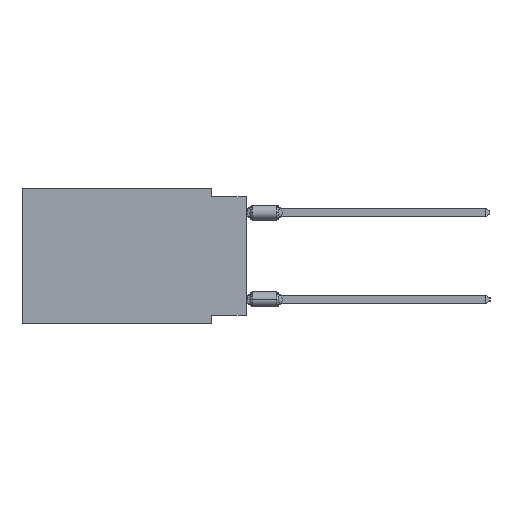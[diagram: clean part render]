
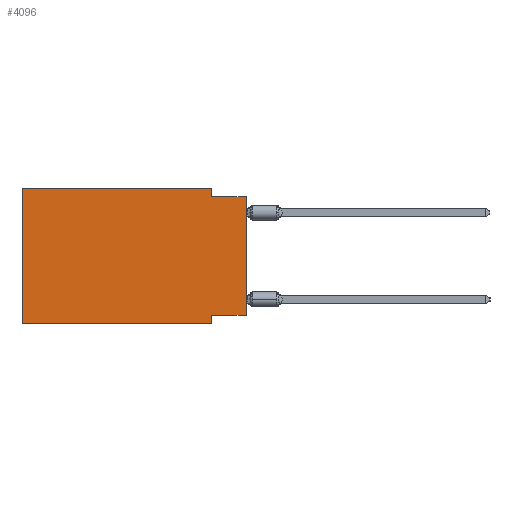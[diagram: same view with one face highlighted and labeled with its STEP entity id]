
A CAD part, left-side view. The second image highlights one B-rep face of the part: STEP entity #4096.
In plain terms, the highlighted planar face has unit normal (-1, 0, 0).
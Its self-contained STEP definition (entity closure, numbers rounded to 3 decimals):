
#33 = CARTESIAN_POINT ( 'NONE',  ( 0., 2.54, -0.635 ) ) ;
#934 = AXIS2_PLACEMENT_3D ( 'NONE', #39811, #10003, #10648 ) ;
#1196 = LINE ( 'NONE', #40220, #36049 ) ;
#1212 = VECTOR ( 'NONE', #21840, 1000. ) ;
#1689 = EDGE_CURVE ( 'NONE', #2483, #50379, #26597, .T. ) ;
#2483 = VERTEX_POINT ( 'NONE', #11028 ) ;
#2522 = EDGE_CURVE ( 'NONE', #21431, #20861, #62807, .T. ) ;
#4096 = ADVANCED_FACE ( 'NONE', ( #26387 ), #54907, .F. ) ;
#5152 = ORIENTED_EDGE ( 'NONE', *, *, #10090, .F. ) ;
#5382 = ORIENTED_EDGE ( 'NONE', *, *, #25717, .F. ) ;
#5768 = VERTEX_POINT ( 'NONE', #33 ) ;
#5859 = EDGE_CURVE ( 'NONE', #32394, #39374, #56073, .T. ) ;
#6676 = VERTEX_POINT ( 'NONE', #11914 ) ;
#7737 = CARTESIAN_POINT ( 'NONE',  ( 0., 16.383, 0. ) ) ;
#10003 = DIRECTION ( 'NONE',  ( 1., 0., 0. ) ) ;
#10090 = EDGE_CURVE ( 'NONE', #32394, #21431, #39053, .T. ) ;
#10648 = DIRECTION ( 'NONE',  ( 0., 0., -1. ) ) ;
#11028 = CARTESIAN_POINT ( 'NONE',  ( 0., 0., -9.271 ) ) ;
#11914 = CARTESIAN_POINT ( 'NONE',  ( 0., 2.54, -9.271 ) ) ;
#12381 = ORIENTED_EDGE ( 'NONE', *, *, #49105, .F. ) ;
#12896 = EDGE_CURVE ( 'NONE', #20861, #5768, #26806, .T. ) ;
#13231 = DIRECTION ( 'NONE',  ( 0., -1., 0. ) ) ;
#16013 = VECTOR ( 'NONE', #50193, 1000. ) ;
#17188 = ORIENTED_EDGE ( 'NONE', *, *, #2522, .F. ) ;
#18573 = DIRECTION ( 'NONE',  ( 0., 0., -1. ) ) ;
#18830 = VECTOR ( 'NONE', #13231, 1000. ) ;
#19734 = ORIENTED_EDGE ( 'NONE', *, *, #1689, .T. ) ;
#20496 = ORIENTED_EDGE ( 'NONE', *, *, #12896, .F. ) ;
#20861 = VERTEX_POINT ( 'NONE', #60413 ) ;
#21067 = VECTOR ( 'NONE', #51495, 1000. ) ;
#21215 = DIRECTION ( 'NONE',  ( 0., 1., 0. ) ) ;
#21431 = VERTEX_POINT ( 'NONE', #33300 ) ;
#21840 = DIRECTION ( 'NONE',  ( 0., -1., 0. ) ) ;
#23506 = CARTESIAN_POINT ( 'NONE',  ( 0., 2.54, -9.906 ) ) ;
#25717 = EDGE_CURVE ( 'NONE', #5768, #50379, #44370, .T. ) ;
#26387 = FACE_OUTER_BOUND ( 'NONE', #40584, .T. ) ;
#26486 = CARTESIAN_POINT ( 'NONE',  ( 0., 2.54, -9.906 ) ) ;
#26581 = DIRECTION ( 'NONE',  ( 0., -1., 0. ) ) ;
#26597 = LINE ( 'NONE', #61659, #21067 ) ;
#26806 = LINE ( 'NONE', #42518, #54850 ) ;
#28279 = VECTOR ( 'NONE', #18573, 1000. ) ;
#29835 = ORIENTED_EDGE ( 'NONE', *, *, #5859, .T. ) ;
#32394 = VERTEX_POINT ( 'NONE', #38095 ) ;
#33300 = CARTESIAN_POINT ( 'NONE',  ( 0., 16.383, 0. ) ) ;
#36049 = VECTOR ( 'NONE', #21215, 1000. ) ;
#38095 = CARTESIAN_POINT ( 'NONE',  ( 0., 16.383, -9.906 ) ) ;
#39053 = LINE ( 'NONE', #43983, #16013 ) ;
#39374 = VERTEX_POINT ( 'NONE', #26486 ) ;
#39416 = CARTESIAN_POINT ( 'NONE',  ( 0., 0., -0.635 ) ) ;
#39811 = CARTESIAN_POINT ( 'NONE',  ( 0., 16.383, 0. ) ) ;
#40220 = CARTESIAN_POINT ( 'NONE',  ( 0., 0., -9.271 ) ) ;
#40584 = EDGE_LOOP ( 'NONE', ( #19734, #5382, #20496, #17188, #5152, #29835, #50986, #12381 ) ) ;
#41870 = DIRECTION ( 'NONE',  ( 0., 0., -1. ) ) ;
#42518 = CARTESIAN_POINT ( 'NONE',  ( 0., 2.54, 0. ) ) ;
#43983 = CARTESIAN_POINT ( 'NONE',  ( 0., 16.383, 0. ) ) ;
#44370 = LINE ( 'NONE', #39416, #18830 ) ;
#49105 = EDGE_CURVE ( 'NONE', #2483, #6676, #1196, .T. ) ;
#49368 = LINE ( 'NONE', #23506, #28279 ) ;
#50193 = DIRECTION ( 'NONE',  ( 0., 0., 1. ) ) ;
#50379 = VERTEX_POINT ( 'NONE', #57584 ) ;
#50986 = ORIENTED_EDGE ( 'NONE', *, *, #56046, .F. ) ;
#51147 = CARTESIAN_POINT ( 'NONE',  ( 0., 16.383, -9.906 ) ) ;
#51495 = DIRECTION ( 'NONE',  ( 0., 0., 1. ) ) ;
#54474 = VECTOR ( 'NONE', #26581, 1000. ) ;
#54850 = VECTOR ( 'NONE', #41870, 1000. ) ;
#54907 = PLANE ( 'NONE',  #934 ) ;
#56046 = EDGE_CURVE ( 'NONE', #6676, #39374, #49368, .T. ) ;
#56073 = LINE ( 'NONE', #51147, #54474 ) ;
#57584 = CARTESIAN_POINT ( 'NONE',  ( 0., 0., -0.635 ) ) ;
#60413 = CARTESIAN_POINT ( 'NONE',  ( 0., 2.54, 0. ) ) ;
#61659 = CARTESIAN_POINT ( 'NONE',  ( 0., 0., 0. ) ) ;
#62807 = LINE ( 'NONE', #7737, #1212 ) ;
